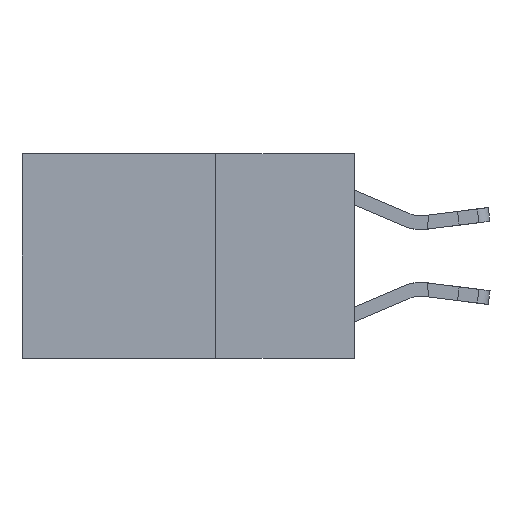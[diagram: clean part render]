
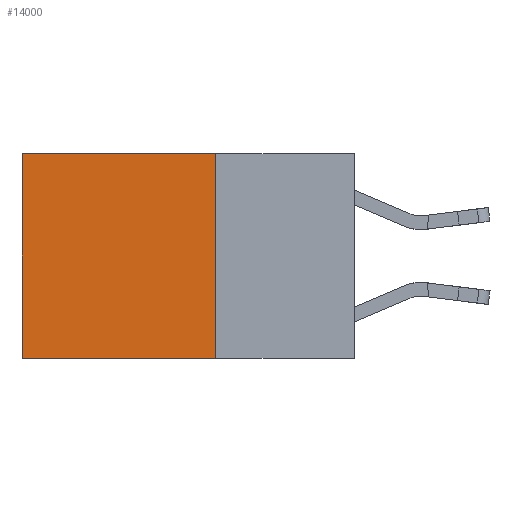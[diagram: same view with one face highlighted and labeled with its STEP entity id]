
A CAD part, left-side view. The second image highlights one B-rep face of the part: STEP entity #14000.
In plain terms, the highlighted planar face has unit normal (-1, 0, 0).
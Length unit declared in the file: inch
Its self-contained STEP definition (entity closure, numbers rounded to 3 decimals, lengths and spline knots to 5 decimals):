
#305 = CARTESIAN_POINT ( 'NONE',  ( 0.2625, 0.6, -0.37 ) ) ;
#1047 = CARTESIAN_POINT ( 'NONE',  ( 0.2625, 0.25, 0. ) ) ;
#2321 = DIRECTION ( 'NONE',  ( 0., 0., -1. ) ) ;
#2523 = CARTESIAN_POINT ( 'NONE',  ( 0.2625, 0.25, 0. ) ) ;
#2538 = EDGE_CURVE ( 'NONE', #14148, #3752, #10048, .T. ) ;
#2554 = ORIENTED_EDGE ( 'NONE', *, *, #3124, .F. ) ;
#2830 = DIRECTION ( 'NONE',  ( 0., 0., -1. ) ) ;
#2899 = CARTESIAN_POINT ( 'NONE',  ( 0.2625, 0.25, -0.37 ) ) ;
#3089 = VECTOR ( 'NONE', #9960, 39.37008 ) ;
#3124 = EDGE_CURVE ( 'NONE', #14148, #6951, #14234, .T. ) ;
#3267 = CARTESIAN_POINT ( 'NONE',  ( 0.2625, 0.6, 0. ) ) ;
#3662 = CARTESIAN_POINT ( 'NONE',  ( 0.2625, 0.25, -0.37 ) ) ;
#3752 = VERTEX_POINT ( 'NONE', #7878 ) ;
#4456 = ORIENTED_EDGE ( 'NONE', *, *, #13526, .F. ) ;
#4509 = VECTOR ( 'NONE', #13116, 39.37008 ) ;
#4811 = PLANE ( 'NONE',  #11532 ) ;
#4918 = DIRECTION ( 'NONE',  ( 0., 1., 0. ) ) ;
#5201 = VECTOR ( 'NONE', #4918, 39.37008 ) ;
#6249 = CARTESIAN_POINT ( 'NONE',  ( 0.2625, 0.25, 0. ) ) ;
#6951 = VERTEX_POINT ( 'NONE', #2899 ) ;
#7729 = EDGE_LOOP ( 'NONE', ( #15898, #4456, #2554, #8454 ) ) ;
#7878 = CARTESIAN_POINT ( 'NONE',  ( 0.2625, 0.6, 0. ) ) ;
#8092 = FACE_OUTER_BOUND ( 'NONE', #7729, .T. ) ;
#8454 = ORIENTED_EDGE ( 'NONE', *, *, #2538, .T. ) ;
#9774 = DIRECTION ( 'NONE',  ( 1., 0., 0. ) ) ;
#9960 = DIRECTION ( 'NONE',  ( 0., 1., 0. ) ) ;
#10048 = LINE ( 'NONE', #2523, #3089 ) ;
#10250 = CARTESIAN_POINT ( 'NONE',  ( 0.2625, 0.25, 0. ) ) ;
#10348 = VERTEX_POINT ( 'NONE', #305 ) ;
#11042 = LINE ( 'NONE', #3267, #4509 ) ;
#11377 = VECTOR ( 'NONE', #2830, 39.37008 ) ;
#11532 = AXIS2_PLACEMENT_3D ( 'NONE', #1047, #9774, #2321 ) ;
#11827 = EDGE_CURVE ( 'NONE', #3752, #10348, #11042, .T. ) ;
#13116 = DIRECTION ( 'NONE',  ( 0., 0., -1. ) ) ;
#13526 = EDGE_CURVE ( 'NONE', #6951, #10348, #14980, .T. ) ;
#14000 = ADVANCED_FACE ( 'NONE', ( #8092 ), #4811, .F. ) ;
#14148 = VERTEX_POINT ( 'NONE', #6249 ) ;
#14234 = LINE ( 'NONE', #10250, #11377 ) ;
#14980 = LINE ( 'NONE', #3662, #5201 ) ;
#15898 = ORIENTED_EDGE ( 'NONE', *, *, #11827, .T. ) ;
